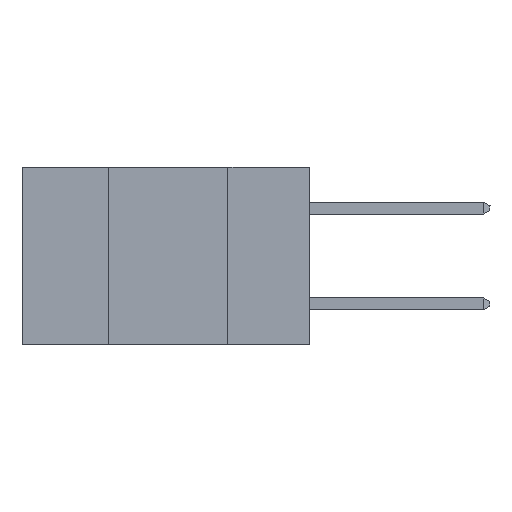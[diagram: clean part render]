
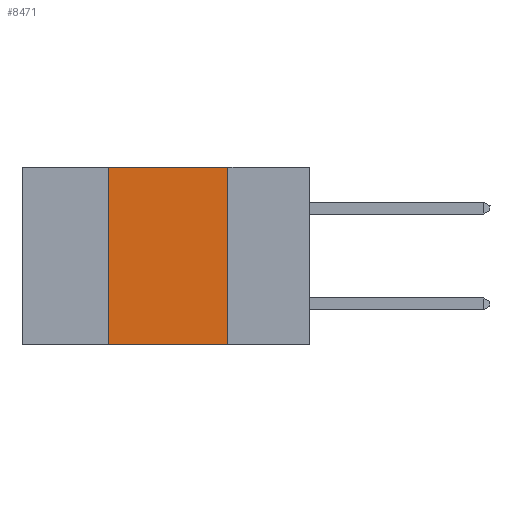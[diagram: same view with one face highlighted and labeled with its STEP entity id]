
A CAD part, left-side view. The second image highlights one B-rep face of the part: STEP entity #8471.
In plain terms, the highlighted planar face has unit normal (-1, 0, 0).
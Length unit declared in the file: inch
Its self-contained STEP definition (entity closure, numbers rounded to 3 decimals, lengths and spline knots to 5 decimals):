
#237 = DIRECTION ( 'NONE',  ( 0., -1., 0. ) ) ;
#254 = FACE_OUTER_BOUND ( 'NONE', #14440, .T. ) ;
#530 = ORIENTED_EDGE ( 'NONE', *, *, #2794, .F. ) ;
#953 = LINE ( 'NONE', #13313, #2267 ) ;
#1237 = VERTEX_POINT ( 'NONE', #11598 ) ;
#2267 = VECTOR ( 'NONE', #10094, 39.37008 ) ;
#2359 = VECTOR ( 'NONE', #5998, 39.37008 ) ;
#2794 = EDGE_CURVE ( 'NONE', #3195, #19310, #9122, .T. ) ;
#3195 = VERTEX_POINT ( 'NONE', #7437 ) ;
#4679 = EDGE_CURVE ( 'NONE', #1237, #19310, #953, .T. ) ;
#5143 = DIRECTION ( 'NONE',  ( 0., 0., 1. ) ) ;
#5998 = DIRECTION ( 'NONE',  ( 0., 0., -1. ) ) ;
#6798 = LINE ( 'NONE', #9906, #13028 ) ;
#6878 = CARTESIAN_POINT ( 'NONE',  ( 0., 0.6, 0. ) ) ;
#7193 = EDGE_CURVE ( 'NONE', #1237, #13122, #6798, .T. ) ;
#7247 = CARTESIAN_POINT ( 'NONE',  ( 0., 0.17, -0.37 ) ) ;
#7437 = CARTESIAN_POINT ( 'NONE',  ( 0., 0.17, 0. ) ) ;
#8459 = PLANE ( 'NONE',  #8520 ) ;
#8471 = ADVANCED_FACE ( 'NONE', ( #254 ), #8459, .F. ) ;
#8520 = AXIS2_PLACEMENT_3D ( 'NONE', #15954, #11467, #9720 ) ;
#9122 = LINE ( 'NONE', #13901, #2359 ) ;
#9720 = DIRECTION ( 'NONE',  ( 0., 0., -1. ) ) ;
#9906 = CARTESIAN_POINT ( 'NONE',  ( 0., 0.42, 0. ) ) ;
#10094 = DIRECTION ( 'NONE',  ( 0., -1., 0. ) ) ;
#11467 = DIRECTION ( 'NONE',  ( 1., 0., 0. ) ) ;
#11598 = CARTESIAN_POINT ( 'NONE',  ( 0., 0.42, -0.37 ) ) ;
#12384 = EDGE_CURVE ( 'NONE', #13122, #3195, #16040, .T. ) ;
#13028 = VECTOR ( 'NONE', #5143, 39.37008 ) ;
#13122 = VERTEX_POINT ( 'NONE', #16651 ) ;
#13313 = CARTESIAN_POINT ( 'NONE',  ( 0., 0.6, -0.37 ) ) ;
#13901 = CARTESIAN_POINT ( 'NONE',  ( 0., 0.17, 0. ) ) ;
#14189 = ORIENTED_EDGE ( 'NONE', *, *, #7193, .F. ) ;
#14440 = EDGE_LOOP ( 'NONE', ( #530, #17495, #14189, #14802 ) ) ;
#14790 = VECTOR ( 'NONE', #237, 39.37008 ) ;
#14802 = ORIENTED_EDGE ( 'NONE', *, *, #4679, .T. ) ;
#15954 = CARTESIAN_POINT ( 'NONE',  ( 0., 0.6, 0. ) ) ;
#16040 = LINE ( 'NONE', #6878, #14790 ) ;
#16651 = CARTESIAN_POINT ( 'NONE',  ( 0., 0.42, 0. ) ) ;
#17495 = ORIENTED_EDGE ( 'NONE', *, *, #12384, .F. ) ;
#19310 = VERTEX_POINT ( 'NONE', #7247 ) ;
